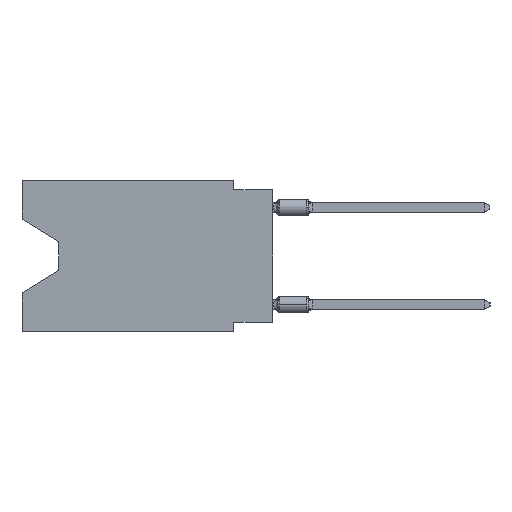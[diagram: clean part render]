
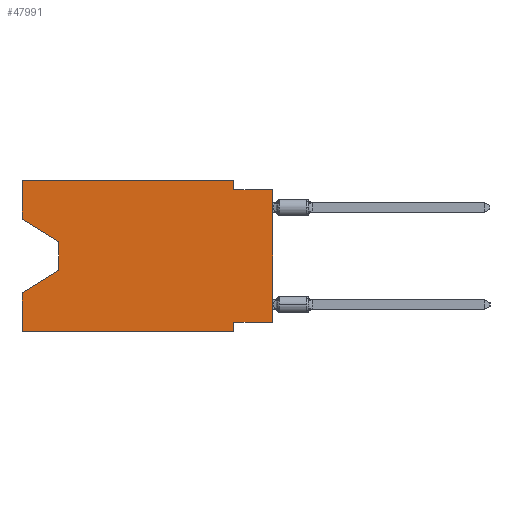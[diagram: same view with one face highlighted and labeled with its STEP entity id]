
A CAD part, left-side view. The second image highlights one B-rep face of the part: STEP entity #47991.
In plain terms, the highlighted planar face has unit normal (-1, 0, 0).
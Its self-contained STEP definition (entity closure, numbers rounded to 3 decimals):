
#130 = EDGE_LOOP ( 'NONE', ( #46608, #22634, #19337, #5782, #7616, #29644, #19509, #17171, #30632, #14424, #26681, #37879 ) ) ;
#658 = LINE ( 'NONE', #39507, #13791 ) ;
#1037 = LINE ( 'NONE', #15971, #5745 ) ;
#1068 = LINE ( 'NONE', #28323, #42038 ) ;
#2088 = EDGE_CURVE ( 'NONE', #50441, #49704, #24163, .T. ) ;
#3575 = VERTEX_POINT ( 'NONE', #38060 ) ;
#3777 = LINE ( 'NONE', #24070, #28012 ) ;
#5141 = VERTEX_POINT ( 'NONE', #17920 ) ;
#5454 = EDGE_CURVE ( 'NONE', #27159, #3575, #658, .T. ) ;
#5745 = VECTOR ( 'NONE', #12869, 1000. ) ;
#5782 = ORIENTED_EDGE ( 'NONE', *, *, #35829, .F. ) ;
#6049 = LINE ( 'NONE', #28936, #6818 ) ;
#6525 = PLANE ( 'NONE',  #15147 ) ;
#6705 = DIRECTION ( 'NONE',  ( 0., 0., -1. ) ) ;
#6818 = VECTOR ( 'NONE', #17888, 1000. ) ;
#7312 = VERTEX_POINT ( 'NONE', #29788 ) ;
#7616 = ORIENTED_EDGE ( 'NONE', *, *, #46046, .T. ) ;
#7698 = CARTESIAN_POINT ( 'NONE',  ( 0., 16.383, -9.906 ) ) ;
#8129 = DIRECTION ( 'NONE',  ( 0., 1., 0. ) ) ;
#8492 = CARTESIAN_POINT ( 'NONE',  ( 0., 16.383, -7.36 ) ) ;
#8563 = CARTESIAN_POINT ( 'NONE',  ( 0., 13.97, -5.893 ) ) ;
#9543 = LINE ( 'NONE', #48638, #23935 ) ;
#9928 = LINE ( 'NONE', #21238, #18068 ) ;
#10132 = CARTESIAN_POINT ( 'NONE',  ( 0., 16.383, 0. ) ) ;
#10770 = EDGE_CURVE ( 'NONE', #20581, #21359, #13230, .T. ) ;
#12200 = LINE ( 'NONE', #23764, #37704 ) ;
#12869 = DIRECTION ( 'NONE',  ( 0., 0., 1. ) ) ;
#13230 = LINE ( 'NONE', #20687, #49474 ) ;
#13791 = VECTOR ( 'NONE', #16338, 1000. ) ;
#14410 = EDGE_CURVE ( 'NONE', #27159, #20847, #12200, .T. ) ;
#14424 = ORIENTED_EDGE ( 'NONE', *, *, #19639, .F. ) ;
#15147 = AXIS2_PLACEMENT_3D ( 'NONE', #10132, #18355, #40744 ) ;
#15971 = CARTESIAN_POINT ( 'NONE',  ( 0., 16.383, 0. ) ) ;
#16222 = DIRECTION ( 'NONE',  ( 0., 0., 1. ) ) ;
#16338 = DIRECTION ( 'NONE',  ( 0., 0., 1. ) ) ;
#17171 = ORIENTED_EDGE ( 'NONE', *, *, #50778, .T. ) ;
#17888 = DIRECTION ( 'NONE',  ( 0., -1., 0. ) ) ;
#17920 = CARTESIAN_POINT ( 'NONE',  ( 0., 2.54, -9.271 ) ) ;
#18068 = VECTOR ( 'NONE', #25341, 1000. ) ;
#18355 = DIRECTION ( 'NONE',  ( 1., 0., 0. ) ) ;
#19109 = EDGE_CURVE ( 'NONE', #7312, #5141, #3777, .T. ) ;
#19337 = ORIENTED_EDGE ( 'NONE', *, *, #2088, .T. ) ;
#19425 = EDGE_CURVE ( 'NONE', #5141, #40967, #1068, .T. ) ;
#19503 = VERTEX_POINT ( 'NONE', #31921 ) ;
#19509 = ORIENTED_EDGE ( 'NONE', *, *, #19109, .F. ) ;
#19639 = EDGE_CURVE ( 'NONE', #19503, #20581, #9543, .T. ) ;
#19717 = DIRECTION ( 'NONE',  ( 0., -1., 0. ) ) ;
#19830 = CARTESIAN_POINT ( 'NONE',  ( 0., 0., 0. ) ) ;
#20581 = VERTEX_POINT ( 'NONE', #38231 ) ;
#20687 = CARTESIAN_POINT ( 'NONE',  ( 0., 0., -0.635 ) ) ;
#20847 = VERTEX_POINT ( 'NONE', #29392 ) ;
#21238 = CARTESIAN_POINT ( 'NONE',  ( 0., 13.97, -4.013 ) ) ;
#21359 = VERTEX_POINT ( 'NONE', #27189 ) ;
#22634 = ORIENTED_EDGE ( 'NONE', *, *, #43596, .T. ) ;
#22636 = VECTOR ( 'NONE', #48091, 1000. ) ;
#23342 = VERTEX_POINT ( 'NONE', #7698 ) ;
#23764 = CARTESIAN_POINT ( 'NONE',  ( 0., 16.383, -2.546 ) ) ;
#23767 = CARTESIAN_POINT ( 'NONE',  ( 0., 2.54, -9.906 ) ) ;
#23905 = CARTESIAN_POINT ( 'NONE',  ( 0., 13.97, -5.893 ) ) ;
#23935 = VECTOR ( 'NONE', #6705, 1000. ) ;
#24070 = CARTESIAN_POINT ( 'NONE',  ( 0., 0., -9.271 ) ) ;
#24163 = LINE ( 'NONE', #23905, #22636 ) ;
#24796 = DIRECTION ( 'NONE',  ( 0., -1., 0. ) ) ;
#25341 = DIRECTION ( 'NONE',  ( 0., 0., -1. ) ) ;
#25964 = VECTOR ( 'NONE', #16222, 1000. ) ;
#26681 = ORIENTED_EDGE ( 'NONE', *, *, #40593, .F. ) ;
#27159 = VERTEX_POINT ( 'NONE', #32251 ) ;
#27189 = CARTESIAN_POINT ( 'NONE',  ( 0., 0., -0.635 ) ) ;
#27805 = DIRECTION ( 'NONE',  ( 0., 0., -1. ) ) ;
#28012 = VECTOR ( 'NONE', #8129, 1000. ) ;
#28323 = CARTESIAN_POINT ( 'NONE',  ( 0., 2.54, -9.906 ) ) ;
#28936 = CARTESIAN_POINT ( 'NONE',  ( 0., 16.383, 0. ) ) ;
#29392 = CARTESIAN_POINT ( 'NONE',  ( 0., 13.97, -4.013 ) ) ;
#29644 = ORIENTED_EDGE ( 'NONE', *, *, #19425, .F. ) ;
#29788 = CARTESIAN_POINT ( 'NONE',  ( 0., 0., -9.271 ) ) ;
#30632 = ORIENTED_EDGE ( 'NONE', *, *, #10770, .F. ) ;
#31921 = CARTESIAN_POINT ( 'NONE',  ( 0., 2.54, 0. ) ) ;
#32251 = CARTESIAN_POINT ( 'NONE',  ( 0., 16.383, -2.546 ) ) ;
#35609 = DIRECTION ( 'NONE',  ( 0., -0.855, -0.519 ) ) ;
#35829 = EDGE_CURVE ( 'NONE', #23342, #49704, #1037, .T. ) ;
#37704 = VECTOR ( 'NONE', #35609, 1000. ) ;
#37879 = ORIENTED_EDGE ( 'NONE', *, *, #5454, .F. ) ;
#38060 = CARTESIAN_POINT ( 'NONE',  ( 0., 16.383, 0. ) ) ;
#38231 = CARTESIAN_POINT ( 'NONE',  ( 0., 2.54, -0.635 ) ) ;
#39507 = CARTESIAN_POINT ( 'NONE',  ( 0., 16.383, 0. ) ) ;
#39625 = VECTOR ( 'NONE', #19717, 1000. ) ;
#40593 = EDGE_CURVE ( 'NONE', #3575, #19503, #6049, .T. ) ;
#40744 = DIRECTION ( 'NONE',  ( 0., 0., -1. ) ) ;
#40967 = VERTEX_POINT ( 'NONE', #23767 ) ;
#40989 = FACE_OUTER_BOUND ( 'NONE', #130, .T. ) ;
#42038 = VECTOR ( 'NONE', #27805, 1000. ) ;
#42877 = LINE ( 'NONE', #50590, #39625 ) ;
#43596 = EDGE_CURVE ( 'NONE', #20847, #50441, #9928, .T. ) ;
#43742 = LINE ( 'NONE', #19830, #25964 ) ;
#46046 = EDGE_CURVE ( 'NONE', #23342, #40967, #42877, .T. ) ;
#46608 = ORIENTED_EDGE ( 'NONE', *, *, #14410, .T. ) ;
#47991 = ADVANCED_FACE ( 'NONE', ( #40989 ), #6525, .F. ) ;
#48091 = DIRECTION ( 'NONE',  ( 0., 0.855, -0.519 ) ) ;
#48638 = CARTESIAN_POINT ( 'NONE',  ( 0., 2.54, 0. ) ) ;
#49474 = VECTOR ( 'NONE', #24796, 1000. ) ;
#49704 = VERTEX_POINT ( 'NONE', #8492 ) ;
#50441 = VERTEX_POINT ( 'NONE', #8563 ) ;
#50590 = CARTESIAN_POINT ( 'NONE',  ( 0., 16.383, -9.906 ) ) ;
#50778 = EDGE_CURVE ( 'NONE', #7312, #21359, #43742, .T. ) ;
